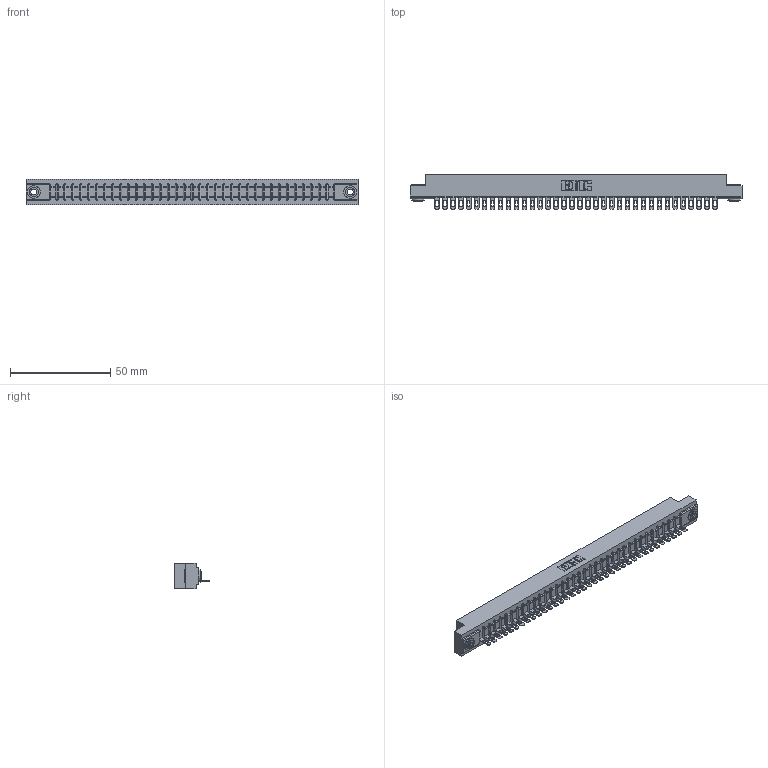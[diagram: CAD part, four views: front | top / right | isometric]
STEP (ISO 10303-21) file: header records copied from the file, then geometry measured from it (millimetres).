
FILE_DESCRIPTION (( 'STEP AP203' ), '1' );
FILE_NAME ('357-036-501-103.STEP', '2019-09-17T06:22:17', ( '' ), ( '' ), 'SwSTEP 2.0', 'SolidWorks 2016', '' );
FILE_SCHEMA (( 'CONFIG_CONTROL_DESIGN' ));
Length unit declared in the file: inch
Products named in the file (4): 345-250-002_345-250-002-102; 307-290-002_501; 357-036-501-103; 307 Part_.156 Dia Mounting Holes
Assembly tree (39 placements, depth 2):
  357-036-501-103
    307 Part_.156 Dia Mounting Holes
    307-290-002_501  x36
    345-250-002_345-250-002-102  x2
Bounding box: 165.66 x 17.42 x 12.7 mm (x, y, z)
Volume: 17715.5 mm3; surface area: 22635.8 mm2
Topology: 39 solids, 39 shells, 2943 faces, 9003 edges, 5898 vertices
Faces by surface type: plane 1678, cylinder 1183, sphere 74, cone 8
Entity records: 33461 total; most frequent: CARTESIAN_POINT 5621, ORIENTED_EDGE 5602, DIRECTION 5483, EDGE_CURVE 2801, VECTOR 2131, LINE 2131, VERTEX_POINT 1814, AXIS2_PLACEMENT_3D 1676
